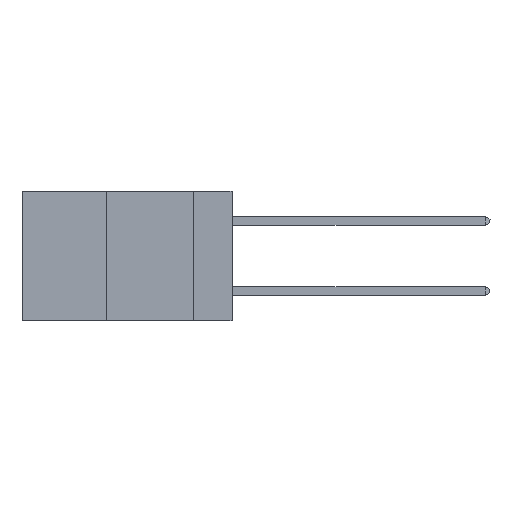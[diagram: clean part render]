
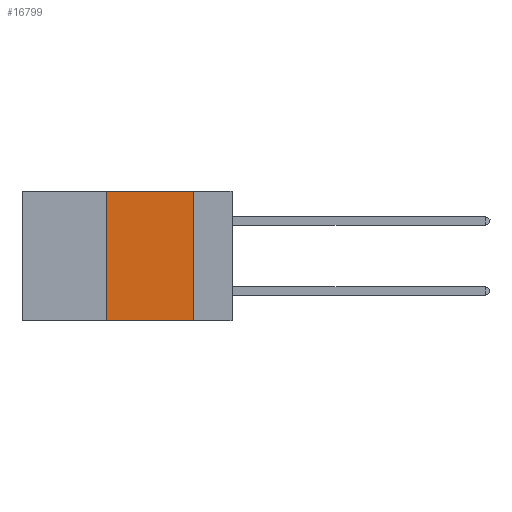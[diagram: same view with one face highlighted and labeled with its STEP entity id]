
A CAD part, left-side view. The second image highlights one B-rep face of the part: STEP entity #16799.
In plain terms, the highlighted planar face has unit normal (-1, 0, 0).
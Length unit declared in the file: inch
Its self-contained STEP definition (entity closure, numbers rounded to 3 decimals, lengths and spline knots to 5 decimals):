
#170 = EDGE_CURVE ( 'NONE', #14481, #10772, #20759, .T. ) ;
#1952 = DIRECTION ( 'NONE',  ( 0., 0., 1. ) ) ;
#2189 = EDGE_CURVE ( 'NONE', #6491, #10772, #12856, .T. ) ;
#2307 = VECTOR ( 'NONE', #21895, 39.37008 ) ;
#3761 = CARTESIAN_POINT ( 'NONE',  ( 0., 0.11, 0. ) ) ;
#6222 = ORIENTED_EDGE ( 'NONE', *, *, #9287, .F. ) ;
#6491 = VERTEX_POINT ( 'NONE', #3761 ) ;
#7045 = DIRECTION ( 'NONE',  ( 0., -1., 0. ) ) ;
#7263 = CARTESIAN_POINT ( 'NONE',  ( 0., 0.6, -0.37 ) ) ;
#7595 = VECTOR ( 'NONE', #7045, 39.37008 ) ;
#8111 = CARTESIAN_POINT ( 'NONE',  ( 0., 0.6, 0. ) ) ;
#9081 = FACE_OUTER_BOUND ( 'NONE', #13125, .T. ) ;
#9287 = EDGE_CURVE ( 'NONE', #31684, #6491, #16257, .T. ) ;
#10772 = VERTEX_POINT ( 'NONE', #26115 ) ;
#12406 = ORIENTED_EDGE ( 'NONE', *, *, #20063, .F. ) ;
#12856 = LINE ( 'NONE', #24452, #31514 ) ;
#13125 = EDGE_LOOP ( 'NONE', ( #20383, #6222, #12406, #15134 ) ) ;
#14481 = VERTEX_POINT ( 'NONE', #31842 ) ;
#15134 = ORIENTED_EDGE ( 'NONE', *, *, #170, .T. ) ;
#16140 = AXIS2_PLACEMENT_3D ( 'NONE', #8111, #25478, #24112 ) ;
#16257 = LINE ( 'NONE', #22471, #2307 ) ;
#16799 = ADVANCED_FACE ( 'NONE', ( #9081 ), #17966, .F. ) ;
#17062 = VECTOR ( 'NONE', #1952, 39.37008 ) ;
#17834 = DIRECTION ( 'NONE',  ( 0., 0., -1. ) ) ;
#17966 = PLANE ( 'NONE',  #16140 ) ;
#18773 = CARTESIAN_POINT ( 'NONE',  ( 0., 0.36, 0. ) ) ;
#20063 = EDGE_CURVE ( 'NONE', #14481, #31684, #23657, .T. ) ;
#20383 = ORIENTED_EDGE ( 'NONE', *, *, #2189, .F. ) ;
#20759 = LINE ( 'NONE', #7263, #7595 ) ;
#21895 = DIRECTION ( 'NONE',  ( 0., -1., 0. ) ) ;
#22471 = CARTESIAN_POINT ( 'NONE',  ( 0., 0.6, 0. ) ) ;
#23657 = LINE ( 'NONE', #18773, #17062 ) ;
#24112 = DIRECTION ( 'NONE',  ( 0., 0., -1. ) ) ;
#24452 = CARTESIAN_POINT ( 'NONE',  ( 0., 0.11, 0. ) ) ;
#25478 = DIRECTION ( 'NONE',  ( 1., 0., 0. ) ) ;
#26115 = CARTESIAN_POINT ( 'NONE',  ( 0., 0.11, -0.37 ) ) ;
#26922 = CARTESIAN_POINT ( 'NONE',  ( 0., 0.36, 0. ) ) ;
#31514 = VECTOR ( 'NONE', #17834, 39.37008 ) ;
#31684 = VERTEX_POINT ( 'NONE', #26922 ) ;
#31842 = CARTESIAN_POINT ( 'NONE',  ( 0., 0.36, -0.37 ) ) ;
